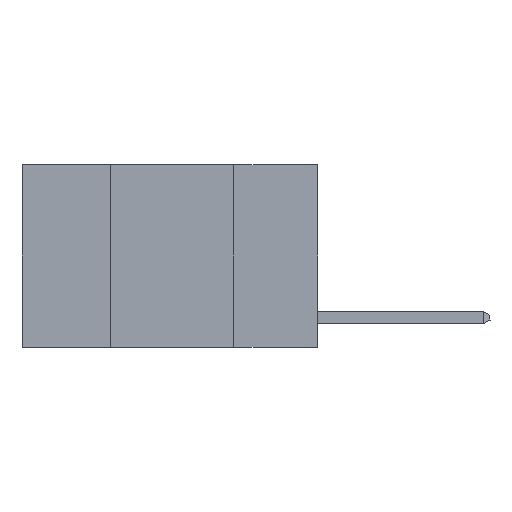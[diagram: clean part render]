
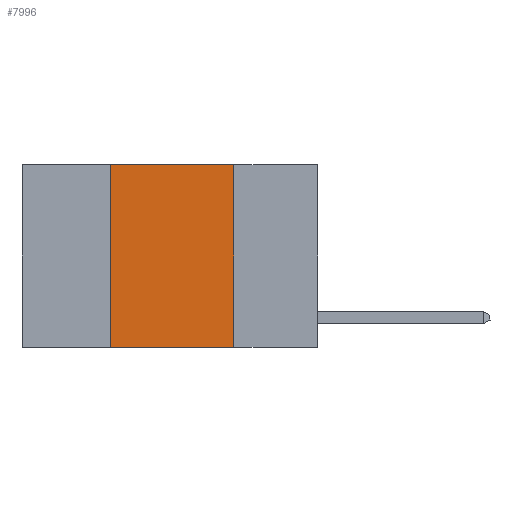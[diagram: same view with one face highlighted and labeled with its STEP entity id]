
A CAD part, left-side view. The second image highlights one B-rep face of the part: STEP entity #7996.
In plain terms, the highlighted planar face has unit normal (-1, 0, 0).
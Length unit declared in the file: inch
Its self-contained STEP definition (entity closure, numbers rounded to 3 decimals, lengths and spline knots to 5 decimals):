
#45 = DIRECTION ( 'NONE',  ( 0., -1., 0. ) ) ;
#217 = PLANE ( 'NONE',  #17556 ) ;
#278 = CARTESIAN_POINT ( 'NONE',  ( 0., 0.6, 0. ) ) ;
#795 = EDGE_CURVE ( 'NONE', #8959, #1287, #10201, .T. ) ;
#1287 = VERTEX_POINT ( 'NONE', #12976 ) ;
#1674 = DIRECTION ( 'NONE',  ( 0., 0., -1. ) ) ;
#2426 = VECTOR ( 'NONE', #2799, 39.37008 ) ;
#2799 = DIRECTION ( 'NONE',  ( 0., 0., 1. ) ) ;
#3214 = VERTEX_POINT ( 'NONE', #11061 ) ;
#3281 = LINE ( 'NONE', #10193, #13919 ) ;
#3457 = EDGE_CURVE ( 'NONE', #8959, #16897, #9733, .T. ) ;
#3850 = EDGE_CURVE ( 'NONE', #1287, #3214, #14599, .T. ) ;
#7024 = CARTESIAN_POINT ( 'NONE',  ( 0., 0.17, -0.37 ) ) ;
#7862 = FACE_OUTER_BOUND ( 'NONE', #10901, .T. ) ;
#7996 = ADVANCED_FACE ( 'NONE', ( #7862 ), #217, .F. ) ;
#8873 = DIRECTION ( 'NONE',  ( 0., -1., 0. ) ) ;
#8959 = VERTEX_POINT ( 'NONE', #13445 ) ;
#9376 = EDGE_CURVE ( 'NONE', #3214, #16897, #3281, .T. ) ;
#9698 = CARTESIAN_POINT ( 'NONE',  ( 0., 0.6, 0. ) ) ;
#9733 = LINE ( 'NONE', #13079, #17169 ) ;
#9934 = DIRECTION ( 'NONE',  ( 1., 0., 0. ) ) ;
#10193 = CARTESIAN_POINT ( 'NONE',  ( 0., 0.17, 0. ) ) ;
#10201 = LINE ( 'NONE', #11590, #2426 ) ;
#10825 = ORIENTED_EDGE ( 'NONE', *, *, #9376, .F. ) ;
#10901 = EDGE_LOOP ( 'NONE', ( #10825, #12888, #12869, #12634 ) ) ;
#11061 = CARTESIAN_POINT ( 'NONE',  ( 0., 0.17, 0. ) ) ;
#11590 = CARTESIAN_POINT ( 'NONE',  ( 0., 0.42, 0. ) ) ;
#11599 = DIRECTION ( 'NONE',  ( 0., 0., -1. ) ) ;
#12634 = ORIENTED_EDGE ( 'NONE', *, *, #3457, .T. ) ;
#12869 = ORIENTED_EDGE ( 'NONE', *, *, #795, .F. ) ;
#12888 = ORIENTED_EDGE ( 'NONE', *, *, #3850, .F. ) ;
#12976 = CARTESIAN_POINT ( 'NONE',  ( 0., 0.42, 0. ) ) ;
#13079 = CARTESIAN_POINT ( 'NONE',  ( 0., 0.6, -0.37 ) ) ;
#13445 = CARTESIAN_POINT ( 'NONE',  ( 0., 0.42, -0.37 ) ) ;
#13919 = VECTOR ( 'NONE', #11599, 39.37008 ) ;
#14599 = LINE ( 'NONE', #9698, #17811 ) ;
#16897 = VERTEX_POINT ( 'NONE', #7024 ) ;
#17169 = VECTOR ( 'NONE', #8873, 39.37008 ) ;
#17556 = AXIS2_PLACEMENT_3D ( 'NONE', #278, #9934, #1674 ) ;
#17811 = VECTOR ( 'NONE', #45, 39.37008 ) ;
